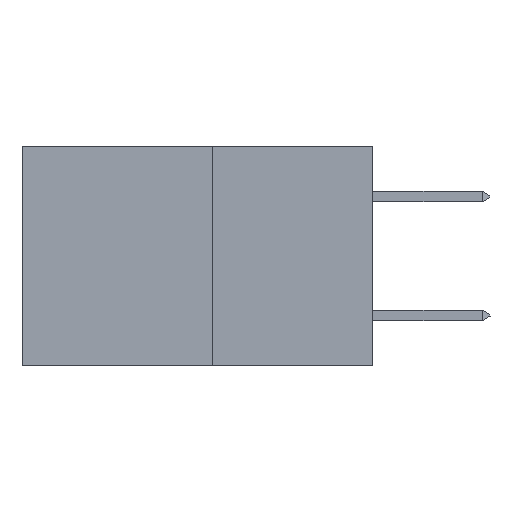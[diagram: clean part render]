
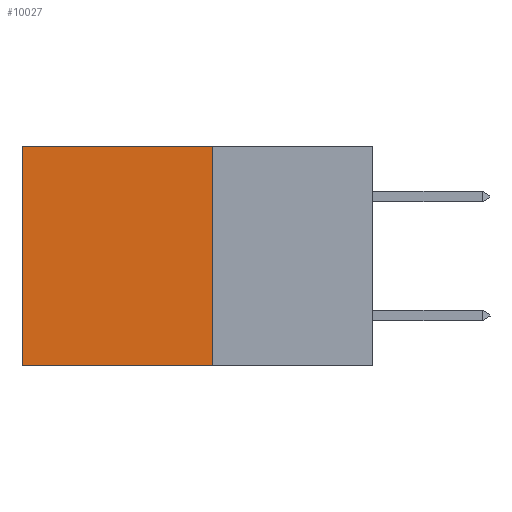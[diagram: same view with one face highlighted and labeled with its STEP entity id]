
A CAD part, left-side view. The second image highlights one B-rep face of the part: STEP entity #10027.
In plain terms, the highlighted planar face has unit normal (-1, 0, 0).
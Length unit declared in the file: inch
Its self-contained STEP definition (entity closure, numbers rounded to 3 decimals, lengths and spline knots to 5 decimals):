
#343 = CARTESIAN_POINT ( 'NONE',  ( 0.277, 0.27, -0.37 ) ) ;
#978 = CARTESIAN_POINT ( 'NONE',  ( 0.277, 0.59, -0.37 ) ) ;
#1060 = LINE ( 'NONE', #4073, #12286 ) ;
#1611 = DIRECTION ( 'NONE',  ( 1., 0., 0. ) ) ;
#2041 = ORIENTED_EDGE ( 'NONE', *, *, #4424, .T. ) ;
#2124 = DIRECTION ( 'NONE',  ( 0., 0., -1. ) ) ;
#2328 = VECTOR ( 'NONE', #2124, 39.37008 ) ;
#2822 = DIRECTION ( 'NONE',  ( 0., 1., 0. ) ) ;
#3351 = VECTOR ( 'NONE', #7098, 39.37008 ) ;
#3821 = VERTEX_POINT ( 'NONE', #3946 ) ;
#3946 = CARTESIAN_POINT ( 'NONE',  ( 0.277, 0.27, -0.37 ) ) ;
#4023 = EDGE_CURVE ( 'NONE', #9010, #7721, #13774, .T. ) ;
#4073 = CARTESIAN_POINT ( 'NONE',  ( 0.277, 0.27, -0.37 ) ) ;
#4424 = EDGE_CURVE ( 'NONE', #7828, #9010, #11622, .T. ) ;
#4761 = CARTESIAN_POINT ( 'NONE',  ( 0.277, 0.27, 0. ) ) ;
#4997 = ORIENTED_EDGE ( 'NONE', *, *, #4023, .T. ) ;
#5516 = AXIS2_PLACEMENT_3D ( 'NONE', #10579, #1611, #9485 ) ;
#5659 = VECTOR ( 'NONE', #2822, 39.37008 ) ;
#7098 = DIRECTION ( 'NONE',  ( 0., 1., 0. ) ) ;
#7124 = FACE_OUTER_BOUND ( 'NONE', #10673, .T. ) ;
#7721 = VERTEX_POINT ( 'NONE', #13473 ) ;
#7828 = VERTEX_POINT ( 'NONE', #4761 ) ;
#8452 = CARTESIAN_POINT ( 'NONE',  ( 0.277, 0.27, 0. ) ) ;
#8595 = DIRECTION ( 'NONE',  ( 0., 0., -1. ) ) ;
#9010 = VERTEX_POINT ( 'NONE', #9278 ) ;
#9278 = CARTESIAN_POINT ( 'NONE',  ( 0.277, 0.59, 0. ) ) ;
#9485 = DIRECTION ( 'NONE',  ( 0., 0., -1. ) ) ;
#9691 = LINE ( 'NONE', #343, #3351 ) ;
#9797 = ORIENTED_EDGE ( 'NONE', *, *, #12045, .F. ) ;
#10027 = ADVANCED_FACE ( 'NONE', ( #7124 ), #12737, .F. ) ;
#10579 = CARTESIAN_POINT ( 'NONE',  ( 0.277, 0.27, -0.37 ) ) ;
#10673 = EDGE_LOOP ( 'NONE', ( #4997, #9797, #14202, #2041 ) ) ;
#11604 = EDGE_CURVE ( 'NONE', #7828, #3821, #1060, .T. ) ;
#11622 = LINE ( 'NONE', #8452, #5659 ) ;
#12045 = EDGE_CURVE ( 'NONE', #3821, #7721, #9691, .T. ) ;
#12286 = VECTOR ( 'NONE', #8595, 39.37008 ) ;
#12737 = PLANE ( 'NONE',  #5516 ) ;
#13473 = CARTESIAN_POINT ( 'NONE',  ( 0.277, 0.59, -0.37 ) ) ;
#13774 = LINE ( 'NONE', #978, #2328 ) ;
#14202 = ORIENTED_EDGE ( 'NONE', *, *, #11604, .F. ) ;
